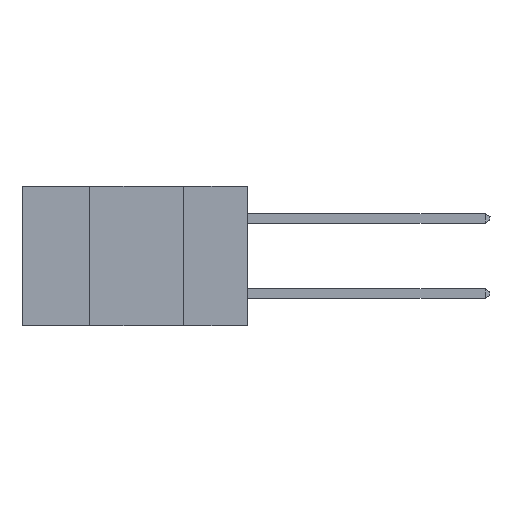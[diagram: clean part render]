
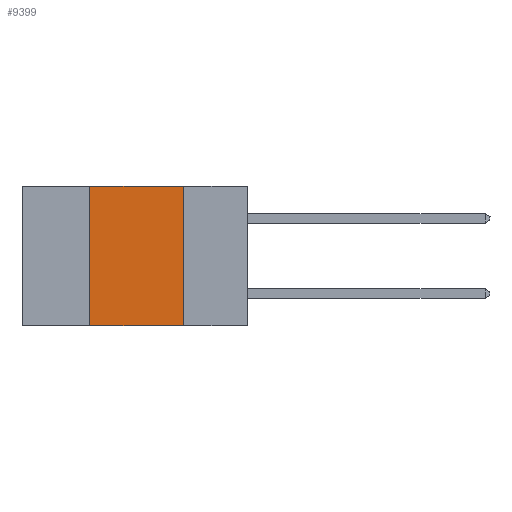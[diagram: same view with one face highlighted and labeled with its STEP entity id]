
A CAD part, left-side view. The second image highlights one B-rep face of the part: STEP entity #9399.
In plain terms, the highlighted planar face has unit normal (-1, 0, 0).
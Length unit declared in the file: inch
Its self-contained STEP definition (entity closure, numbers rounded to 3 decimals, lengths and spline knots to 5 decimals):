
#130 = VECTOR ( 'NONE', #869, 39.37008 ) ;
#481 = ORIENTED_EDGE ( 'NONE', *, *, #3168, .F. ) ;
#869 = DIRECTION ( 'NONE',  ( 0., -1., 0. ) ) ;
#923 = LINE ( 'NONE', #14289, #1542 ) ;
#1218 = VERTEX_POINT ( 'NONE', #9771 ) ;
#1542 = VECTOR ( 'NONE', #14212, 39.37008 ) ;
#1604 = VERTEX_POINT ( 'NONE', #4821 ) ;
#1734 = LINE ( 'NONE', #6522, #9643 ) ;
#1959 = FACE_OUTER_BOUND ( 'NONE', #13898, .T. ) ;
#3148 = EDGE_CURVE ( 'NONE', #9899, #6906, #12583, .T. ) ;
#3168 = EDGE_CURVE ( 'NONE', #9899, #1218, #1734, .T. ) ;
#3392 = PLANE ( 'NONE',  #11267 ) ;
#3609 = LINE ( 'NONE', #8222, #9175 ) ;
#3755 = ORIENTED_EDGE ( 'NONE', *, *, #6213, .F. ) ;
#4322 = DIRECTION ( 'NONE',  ( 0., 0., -1. ) ) ;
#4821 = CARTESIAN_POINT ( 'NONE',  ( 0., 0.17, 0. ) ) ;
#6213 = EDGE_CURVE ( 'NONE', #1218, #1604, #3609, .T. ) ;
#6391 = CARTESIAN_POINT ( 'NONE',  ( 0., 0.17, -0.37 ) ) ;
#6522 = CARTESIAN_POINT ( 'NONE',  ( 0., 0.42, -0.37 ) ) ;
#6906 = VERTEX_POINT ( 'NONE', #6391 ) ;
#7011 = ORIENTED_EDGE ( 'NONE', *, *, #14369, .F. ) ;
#7911 = CARTESIAN_POINT ( 'NONE',  ( 0., 0.6, -0.37 ) ) ;
#7992 = DIRECTION ( 'NONE',  ( 1., 0., 0. ) ) ;
#8074 = CARTESIAN_POINT ( 'NONE',  ( 0., 0.6, 0. ) ) ;
#8222 = CARTESIAN_POINT ( 'NONE',  ( 0., 0.6, 0. ) ) ;
#8373 = DIRECTION ( 'NONE',  ( 0., -1., 0. ) ) ;
#9175 = VECTOR ( 'NONE', #8373, 39.37008 ) ;
#9399 = ADVANCED_FACE ( 'NONE', ( #1959 ), #3392, .F. ) ;
#9643 = VECTOR ( 'NONE', #14452, 39.37008 ) ;
#9771 = CARTESIAN_POINT ( 'NONE',  ( 0., 0.42, 0. ) ) ;
#9899 = VERTEX_POINT ( 'NONE', #13313 ) ;
#10278 = ORIENTED_EDGE ( 'NONE', *, *, #3148, .T. ) ;
#11267 = AXIS2_PLACEMENT_3D ( 'NONE', #8074, #7992, #4322 ) ;
#12583 = LINE ( 'NONE', #7911, #130 ) ;
#13313 = CARTESIAN_POINT ( 'NONE',  ( 0., 0.42, -0.37 ) ) ;
#13898 = EDGE_LOOP ( 'NONE', ( #7011, #3755, #481, #10278 ) ) ;
#14212 = DIRECTION ( 'NONE',  ( 0., 0., -1. ) ) ;
#14289 = CARTESIAN_POINT ( 'NONE',  ( 0., 0.17, -0.37 ) ) ;
#14369 = EDGE_CURVE ( 'NONE', #1604, #6906, #923, .T. ) ;
#14452 = DIRECTION ( 'NONE',  ( 0., 0., 1. ) ) ;
